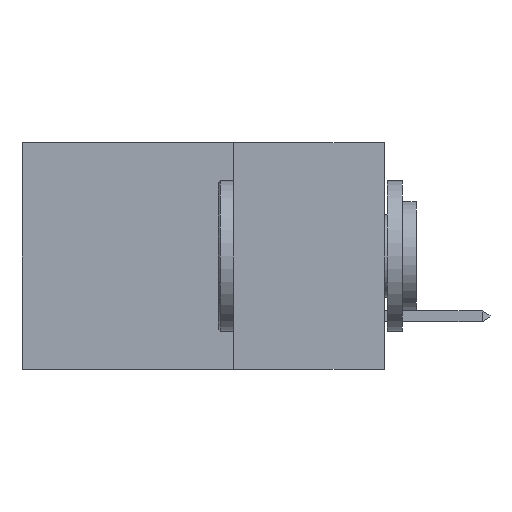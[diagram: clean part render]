
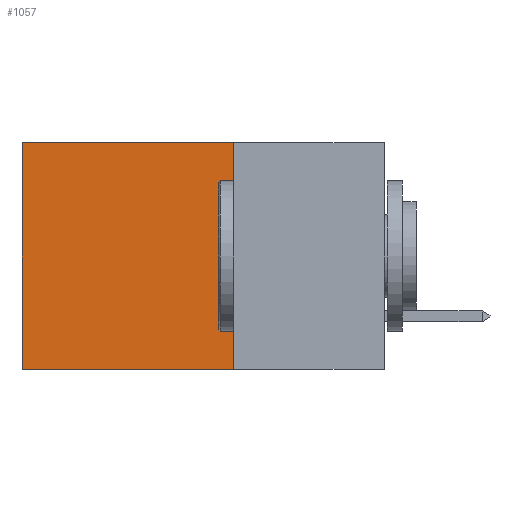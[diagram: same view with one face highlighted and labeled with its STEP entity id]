
A CAD part, left-side view. The second image highlights one B-rep face of the part: STEP entity #1057.
In plain terms, the highlighted planar face has unit normal (-1, 0, 0).
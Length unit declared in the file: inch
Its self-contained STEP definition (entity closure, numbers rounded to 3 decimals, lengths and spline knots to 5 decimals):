
#392 = CARTESIAN_POINT ( 'NONE',  ( 0.2875, 0.6, -0.375 ) ) ;
#460 = CARTESIAN_POINT ( 'NONE',  ( 0.2875, 0.6, 0. ) ) ;
#934 = LINE ( 'NONE', #11517, #11199 ) ;
#1057 = ADVANCED_FACE ( 'NONE', ( #9010 ), #13507, .F. ) ;
#2725 = DIRECTION ( 'NONE',  ( 0., 1., 0. ) ) ;
#2775 = DIRECTION ( 'NONE',  ( 0., 1., 0. ) ) ;
#3357 = VERTEX_POINT ( 'NONE', #5081 ) ;
#3928 = CARTESIAN_POINT ( 'NONE',  ( 0.2875, 0.25, -0.375 ) ) ;
#4562 = VERTEX_POINT ( 'NONE', #392 ) ;
#4710 = DIRECTION ( 'NONE',  ( 0., 0., -1. ) ) ;
#4782 = DIRECTION ( 'NONE',  ( 1., 0., 0. ) ) ;
#4907 = ORIENTED_EDGE ( 'NONE', *, *, #5362, .F. ) ;
#5081 = CARTESIAN_POINT ( 'NONE',  ( 0.2875, 0.25, 0. ) ) ;
#5236 = DIRECTION ( 'NONE',  ( 0., 0., -1. ) ) ;
#5362 = EDGE_CURVE ( 'NONE', #5394, #4562, #6902, .T. ) ;
#5394 = VERTEX_POINT ( 'NONE', #9430 ) ;
#5500 = LINE ( 'NONE', #9804, #6690 ) ;
#6690 = VECTOR ( 'NONE', #7696, 39.37008 ) ;
#6801 = VECTOR ( 'NONE', #2725, 39.37008 ) ;
#6884 = LINE ( 'NONE', #12374, #8467 ) ;
#6902 = LINE ( 'NONE', #3928, #6801 ) ;
#7084 = EDGE_CURVE ( 'NONE', #3357, #9240, #6884, .T. ) ;
#7227 = EDGE_LOOP ( 'NONE', ( #10739, #4907, #8436, #7977 ) ) ;
#7615 = EDGE_CURVE ( 'NONE', #9240, #4562, #5500, .T. ) ;
#7696 = DIRECTION ( 'NONE',  ( 0., 0., -1. ) ) ;
#7977 = ORIENTED_EDGE ( 'NONE', *, *, #7084, .T. ) ;
#8247 = EDGE_CURVE ( 'NONE', #3357, #5394, #934, .T. ) ;
#8436 = ORIENTED_EDGE ( 'NONE', *, *, #8247, .F. ) ;
#8467 = VECTOR ( 'NONE', #2775, 39.37008 ) ;
#9010 = FACE_OUTER_BOUND ( 'NONE', #7227, .T. ) ;
#9240 = VERTEX_POINT ( 'NONE', #460 ) ;
#9430 = CARTESIAN_POINT ( 'NONE',  ( 0.2875, 0.25, -0.375 ) ) ;
#9680 = AXIS2_PLACEMENT_3D ( 'NONE', #12383, #4782, #4710 ) ;
#9804 = CARTESIAN_POINT ( 'NONE',  ( 0.2875, 0.6, -0.375 ) ) ;
#10739 = ORIENTED_EDGE ( 'NONE', *, *, #7615, .T. ) ;
#11199 = VECTOR ( 'NONE', #5236, 39.37008 ) ;
#11517 = CARTESIAN_POINT ( 'NONE',  ( 0.2875, 0.25, -0.375 ) ) ;
#12374 = CARTESIAN_POINT ( 'NONE',  ( 0.2875, 0.25, 0. ) ) ;
#12383 = CARTESIAN_POINT ( 'NONE',  ( 0.2875, 0.25, -0.375 ) ) ;
#13507 = PLANE ( 'NONE',  #9680 ) ;
